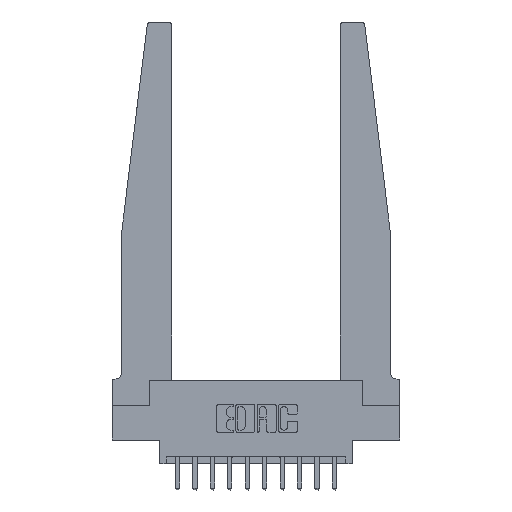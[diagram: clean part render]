
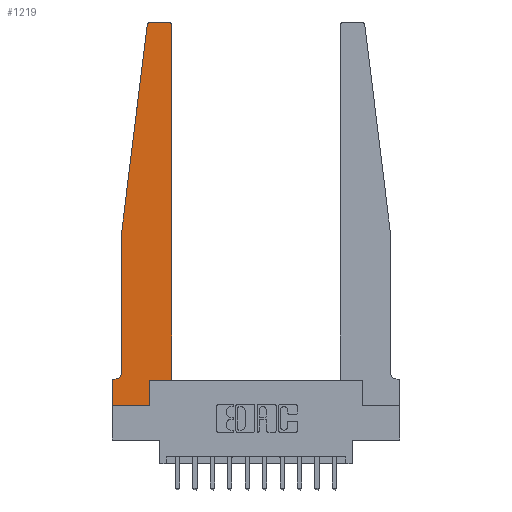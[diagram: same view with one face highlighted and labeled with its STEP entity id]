
A CAD part, top view. The second image highlights one B-rep face of the part: STEP entity #1219.
In plain terms, the highlighted planar face has unit normal (0, 0, 1).
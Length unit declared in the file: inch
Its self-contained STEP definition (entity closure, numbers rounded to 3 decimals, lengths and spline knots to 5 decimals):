
#130 = EDGE_LOOP ( 'NONE', ( #9537, #9034, #2752, #8552, #11899, #624, #12211, #9832, #1771, #14340, #9501, #4694 ) ) ;
#205 = VECTOR ( 'NONE', #7853, 39.37008 ) ;
#624 = ORIENTED_EDGE ( 'NONE', *, *, #10693, .T. ) ;
#824 = DIRECTION ( 'NONE',  ( 0., -1., 0. ) ) ;
#914 = CARTESIAN_POINT ( 'NONE',  ( 0., 0., 0.37 ) ) ;
#957 = LINE ( 'NONE', #5985, #13061 ) ;
#1143 = CARTESIAN_POINT ( 'NONE',  ( 0.395, 2.75, 0.37 ) ) ;
#1219 = ADVANCED_FACE ( 'NONE', ( #11044 ), #9564, .T. ) ;
#1383 = CARTESIAN_POINT ( 'NONE',  ( 0.425, 0.18, 0.37 ) ) ;
#1461 = LINE ( 'NONE', #1383, #10417 ) ;
#1771 = ORIENTED_EDGE ( 'NONE', *, *, #14556, .T. ) ;
#1809 = EDGE_CURVE ( 'NONE', #11548, #10599, #3576, .T. ) ;
#1820 = VECTOR ( 'NONE', #11185, 39.37008 ) ;
#2080 = AXIS2_PLACEMENT_3D ( 'NONE', #11021, #4409, #12334 ) ;
#2228 = DIRECTION ( 'NONE',  ( -1., 0., 0. ) ) ;
#2348 = CARTESIAN_POINT ( 'NONE',  ( 0.2605, 0., 0.37 ) ) ;
#2372 = DIRECTION ( 'NONE',  ( -0.122, -0.992, 0. ) ) ;
#2374 = DIRECTION ( 'NONE',  ( 0., 0., 1. ) ) ;
#2752 = ORIENTED_EDGE ( 'NONE', *, *, #15316, .T. ) ;
#2910 = VECTOR ( 'NONE', #2228, 39.37008 ) ;
#3047 = VECTOR ( 'NONE', #2372, 39.37008 ) ;
#3225 = CARTESIAN_POINT ( 'NONE',  ( 0.015, 0.1875, 0.37 ) ) ;
#3330 = DIRECTION ( 'NONE',  ( 1., 0., 0. ) ) ;
#3491 = DIRECTION ( 'NONE',  ( 0., 1., 0. ) ) ;
#3576 = LINE ( 'NONE', #7567, #1820 ) ;
#4409 = DIRECTION ( 'NONE',  ( 0., 0., 1. ) ) ;
#4486 = VERTEX_POINT ( 'NONE', #4621 ) ;
#4555 = CARTESIAN_POINT ( 'NONE',  ( 0., 0., 0.37 ) ) ;
#4621 = CARTESIAN_POINT ( 'NONE',  ( 0., 0.1875, 0.37 ) ) ;
#4694 = ORIENTED_EDGE ( 'NONE', *, *, #5185, .T. ) ;
#4762 = VERTEX_POINT ( 'NONE', #3225 ) ;
#5185 = EDGE_CURVE ( 'NONE', #6946, #15246, #5235, .T. ) ;
#5235 = CIRCLE ( 'NONE', #2080, 0.03 ) ;
#5644 = EDGE_CURVE ( 'NONE', #7341, #8152, #6311, .T. ) ;
#5818 = CARTESIAN_POINT ( 'NONE',  ( 0.015, 0.2375, 0.37 ) ) ;
#5985 = CARTESIAN_POINT ( 'NONE',  ( 0.2605, 0.18, 0.37 ) ) ;
#6114 = CARTESIAN_POINT ( 'NONE',  ( 0.25, 2.75, 0.37 ) ) ;
#6311 = CIRCLE ( 'NONE', #14462, 0.03 ) ;
#6582 = EDGE_CURVE ( 'NONE', #15246, #7341, #12459, .T. ) ;
#6946 = VERTEX_POINT ( 'NONE', #11753 ) ;
#6960 = AXIS2_PLACEMENT_3D ( 'NONE', #8333, #2374, #12126 ) ;
#7086 = CARTESIAN_POINT ( 'NONE',  ( 0.065, 1.25, 0.37 ) ) ;
#7187 = EDGE_CURVE ( 'NONE', #14870, #14448, #9440, .T. ) ;
#7199 = CIRCLE ( 'NONE', #13506, 0.05 ) ;
#7341 = VERTEX_POINT ( 'NONE', #14777 ) ;
#7361 = CARTESIAN_POINT ( 'NONE',  ( 0.425, 0.18, 0.37 ) ) ;
#7567 = CARTESIAN_POINT ( 'NONE',  ( 0.425, 0.18, 0.37 ) ) ;
#7853 = DIRECTION ( 'NONE',  ( -1., 0., 0. ) ) ;
#8152 = VERTEX_POINT ( 'NONE', #13507 ) ;
#8333 = CARTESIAN_POINT ( 'NONE',  ( 0., 0.1875, 0.37 ) ) ;
#8372 = DIRECTION ( 'NONE',  ( 1., 0., 0. ) ) ;
#8552 = ORIENTED_EDGE ( 'NONE', *, *, #13949, .T. ) ;
#8649 = LINE ( 'NONE', #13500, #3047 ) ;
#8888 = DIRECTION ( 'NONE',  ( 0., 1., 0. ) ) ;
#9034 = ORIENTED_EDGE ( 'NONE', *, *, #5644, .T. ) ;
#9077 = VECTOR ( 'NONE', #12206, 39.37008 ) ;
#9244 = LINE ( 'NONE', #14253, #205 ) ;
#9440 = LINE ( 'NONE', #4555, #15912 ) ;
#9501 = ORIENTED_EDGE ( 'NONE', *, *, #14115, .T. ) ;
#9537 = ORIENTED_EDGE ( 'NONE', *, *, #6582, .T. ) ;
#9564 = PLANE ( 'NONE',  #6960 ) ;
#9832 = ORIENTED_EDGE ( 'NONE', *, *, #7187, .T. ) ;
#10417 = VECTOR ( 'NONE', #8888, 39.37008 ) ;
#10599 = VERTEX_POINT ( 'NONE', #7361 ) ;
#10678 = DIRECTION ( 'NONE',  ( 0., 0., 1. ) ) ;
#10693 = EDGE_CURVE ( 'NONE', #4762, #4486, #9244, .T. ) ;
#10859 = DIRECTION ( 'NONE',  ( 0., 0., -1. ) ) ;
#10932 = DIRECTION ( 'NONE',  ( -1., 0., 0. ) ) ;
#11021 = CARTESIAN_POINT ( 'NONE',  ( 0.395, 2.72, 0.37 ) ) ;
#11044 = FACE_OUTER_BOUND ( 'NONE', #130, .T. ) ;
#11185 = DIRECTION ( 'NONE',  ( 1., 0., 0. ) ) ;
#11195 = LINE ( 'NONE', #7086, #16189 ) ;
#11305 = EDGE_CURVE ( 'NONE', #14818, #4762, #7199, .T. ) ;
#11548 = VERTEX_POINT ( 'NONE', #15035 ) ;
#11729 = VERTEX_POINT ( 'NONE', #16008 ) ;
#11753 = CARTESIAN_POINT ( 'NONE',  ( 0.425, 2.72, 0.37 ) ) ;
#11899 = ORIENTED_EDGE ( 'NONE', *, *, #11305, .T. ) ;
#12126 = DIRECTION ( 'NONE',  ( 1., 0., 0. ) ) ;
#12206 = DIRECTION ( 'NONE',  ( 0., -1., 0. ) ) ;
#12211 = ORIENTED_EDGE ( 'NONE', *, *, #13424, .T. ) ;
#12334 = DIRECTION ( 'NONE',  ( 1., 0., 0. ) ) ;
#12459 = LINE ( 'NONE', #6114, #2910 ) ;
#13061 = VECTOR ( 'NONE', #3491, 39.37008 ) ;
#13424 = EDGE_CURVE ( 'NONE', #4486, #14870, #16147, .T. ) ;
#13500 = CARTESIAN_POINT ( 'NONE',  ( 0.065, 1.25, 0.37 ) ) ;
#13506 = AXIS2_PLACEMENT_3D ( 'NONE', #5818, #10859, #10932 ) ;
#13507 = CARTESIAN_POINT ( 'NONE',  ( 0.24675, 2.72367, 0.37 ) ) ;
#13949 = EDGE_CURVE ( 'NONE', #11729, #14818, #11195, .T. ) ;
#14115 = EDGE_CURVE ( 'NONE', #10599, #6946, #1461, .T. ) ;
#14253 = CARTESIAN_POINT ( 'NONE',  ( 0.065, 0.1875, 0.37 ) ) ;
#14340 = ORIENTED_EDGE ( 'NONE', *, *, #1809, .T. ) ;
#14448 = VERTEX_POINT ( 'NONE', #2348 ) ;
#14462 = AXIS2_PLACEMENT_3D ( 'NONE', #15862, #10678, #8372 ) ;
#14556 = EDGE_CURVE ( 'NONE', #14448, #11548, #957, .T. ) ;
#14777 = CARTESIAN_POINT ( 'NONE',  ( 0.27653, 2.75, 0.37 ) ) ;
#14818 = VERTEX_POINT ( 'NONE', #14999 ) ;
#14824 = CARTESIAN_POINT ( 'NONE',  ( 0., 0., 0.37 ) ) ;
#14870 = VERTEX_POINT ( 'NONE', #914 ) ;
#14999 = CARTESIAN_POINT ( 'NONE',  ( 0.065, 0.2375, 0.37 ) ) ;
#15035 = CARTESIAN_POINT ( 'NONE',  ( 0.2605, 0.18, 0.37 ) ) ;
#15246 = VERTEX_POINT ( 'NONE', #1143 ) ;
#15316 = EDGE_CURVE ( 'NONE', #8152, #11729, #8649, .T. ) ;
#15862 = CARTESIAN_POINT ( 'NONE',  ( 0.27653, 2.72, 0.37 ) ) ;
#15912 = VECTOR ( 'NONE', #3330, 39.37008 ) ;
#16008 = CARTESIAN_POINT ( 'NONE',  ( 0.065, 1.25, 0.37 ) ) ;
#16147 = LINE ( 'NONE', #14824, #9077 ) ;
#16189 = VECTOR ( 'NONE', #824, 39.37008 ) ;
